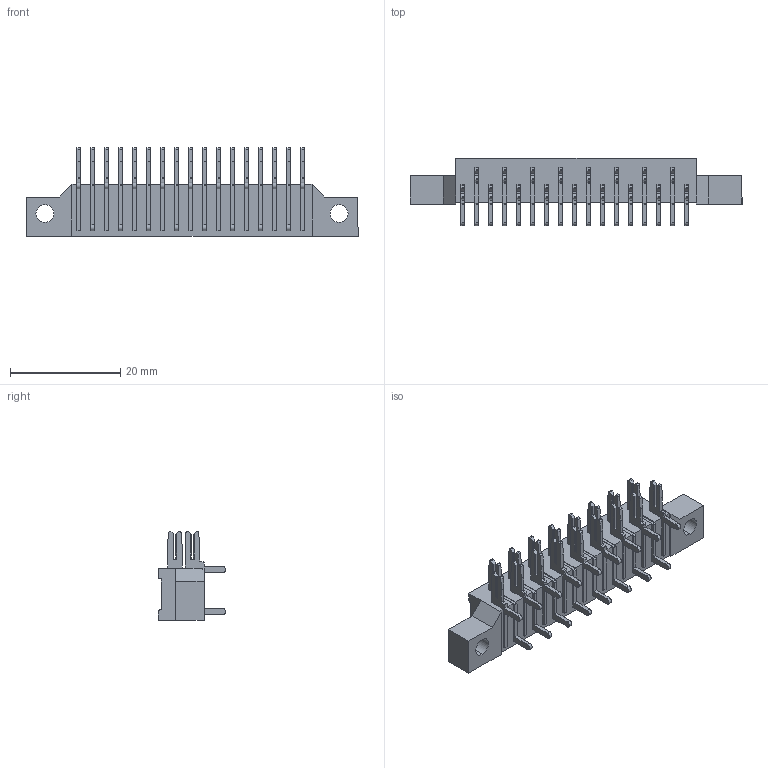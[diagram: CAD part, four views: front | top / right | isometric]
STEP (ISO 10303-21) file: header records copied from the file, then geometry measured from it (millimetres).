
FILE_DESCRIPTION (( 'STEP AP203' ), '1' );
FILE_NAME ('421-017-521-102.STEP', '2019-11-28T19:29:23', ( '' ), ( '' ), 'SwSTEP 2.0', 'SolidWorks 2016', '' );
FILE_SCHEMA (( 'CONFIG_CONTROL_DESIGN' ));
Length unit declared in the file: inch
Products named in the file (4): 421-290-002_121; 421-290-001_121; 421-017-521-102; 421 Part_17
Assembly tree (18 placements, depth 2):
  421-017-521-102
    421 Part_17
    421-290-001_121  x8
    421-290-002_121  x9
Bounding box: 60.2 x 12.17 x 16.05 mm (x, y, z)
Volume: 3897.4 mm3; surface area: 6160.2 mm2
Topology: 18 solids, 18 shells, 638 faces, 1784 edges, 1188 vertices
Faces by surface type: plane 508, cylinder 130
Entity records: 8368 total; most frequent: CARTESIAN_POINT 1345, ORIENTED_EDGE 1312, DIRECTION 1272, EDGE_CURVE 656, VECTOR 546, LINE 546, VERTEX_POINT 436, AXIS2_PLACEMENT_3D 363
